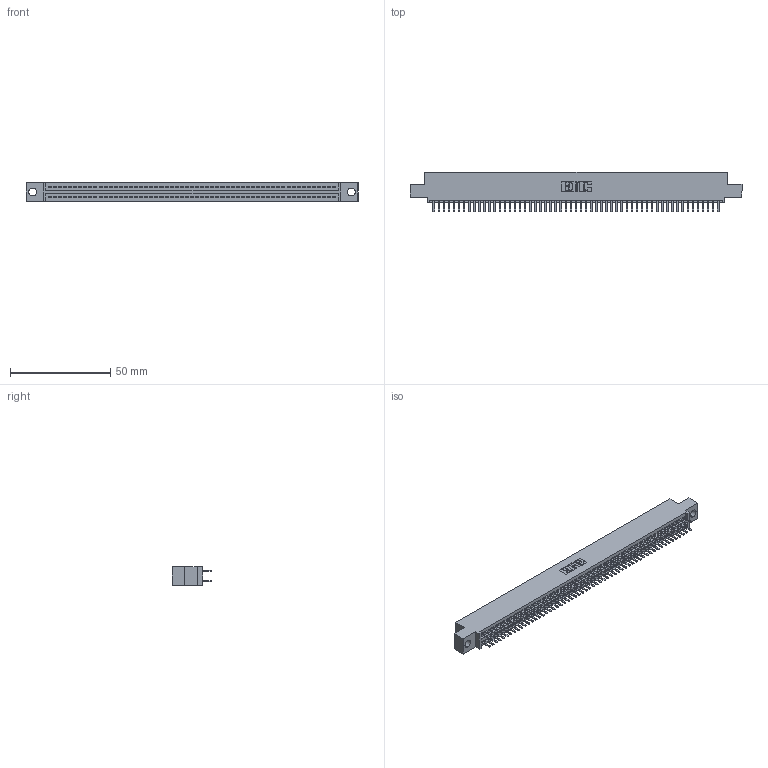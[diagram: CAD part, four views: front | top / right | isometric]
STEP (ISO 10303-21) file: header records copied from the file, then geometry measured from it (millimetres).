
FILE_DESCRIPTION (( 'STEP AP203' ), '1' );
FILE_NAME ('395-114-520-504.STEP', '2021-06-17T18:39:17', ( '' ), ( '' ), 'SwSTEP 2.0', 'SolidWorks 2020', '' );
FILE_SCHEMA (( 'CONFIG_CONTROL_DESIGN' ));
Length unit declared in the file: inch
Products named in the file (3): 345 Part_0.110 Offset - 0.156 Dia-TI; 345-292-001_345-293-120; 395-114-520-504
Assembly tree (115 placements, depth 2):
  395-114-520-504
    345 Part_0.110 Offset - 0.156 Dia-TI
    345-292-001_345-293-120  x114
Bounding box: 165.99 x 19.68 x 9.4 mm (x, y, z)
Volume: 16034.1 mm3; surface area: 23829.5 mm2
Topology: 115 solids, 115 shells, 6300 faces, 18287 edges, 11886 vertices
Faces by surface type: plane 4088, cylinder 2212
Entity records: 43369 total; most frequent: CARTESIAN_POINT 7274, ORIENTED_EDGE 7194, DIRECTION 6381, EDGE_CURVE 3597, VECTOR 3233, LINE 3233, VERTEX_POINT 2394, AXIS2_PLACEMENT_3D 1574
